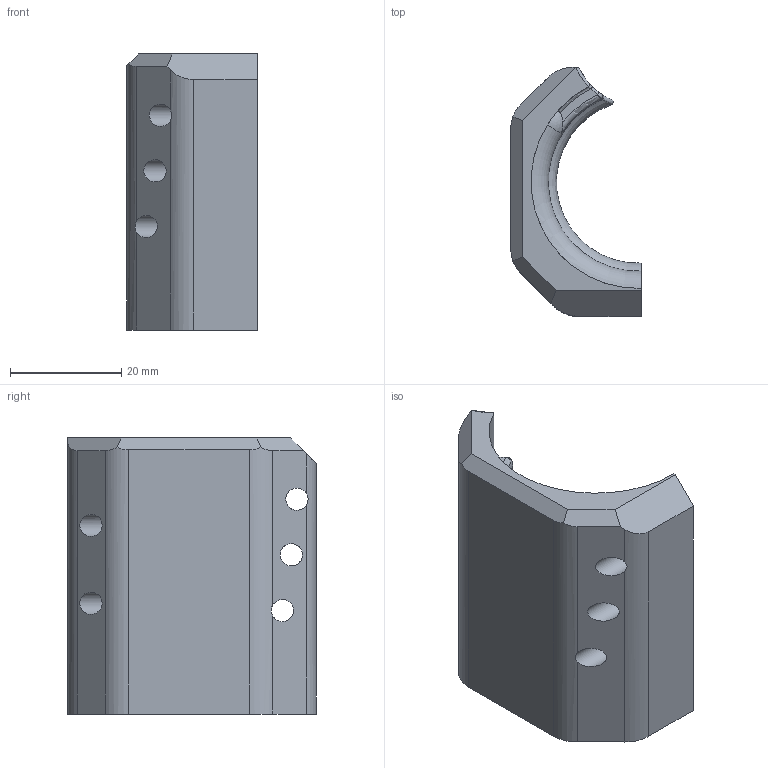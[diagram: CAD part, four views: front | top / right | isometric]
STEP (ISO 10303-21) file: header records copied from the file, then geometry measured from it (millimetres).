
FILE_DESCRIPTION(/* description */ (''),/* implementation_level */ '2;1');
FILE_NAME(/* name */ 'Barrel Mount Left Rev7.stp',/* time_stamp */ '2022-03-16T22:00:56-05:00',/* author */ ('johne'),/* organization */ (''),/* preprocessor_version */ 'ST-DEVELOPER v18.1',/* originating_system */ 'Autodesk Inventor 2020',/* authorisation */ '');
FILE_SCHEMA (('AUTOMOTIVE_DESIGN { 1 0 10303 214 3 1 1 }'));
Length unit declared in the file: millimetre
Products named in the file (1): Barrel Mount Right Rev7
Bounding box: 23.44 x 44.67 x 49.6 mm (x, y, z)
Volume: 19944 mm3; surface area: 8013.7 mm2
Topology: 1 solids, 1 shells, 59 faces, 163 edges, 105 vertices
Faces by surface type: cylinder 18, plane 17, torus 12, bspline 10, sphere 2
Full cylindrical faces by diameter (mm): 4 x5
Entity records: 2536 total; most frequent: CARTESIAN_POINT 1013, ORIENTED_EDGE 324, DIRECTION 301, EDGE_CURVE 162, AXIS2_PLACEMENT_3D 125, VERTEX_POINT 105, EDGE_LOOP 65, FACE_OUTER_BOUND 59
